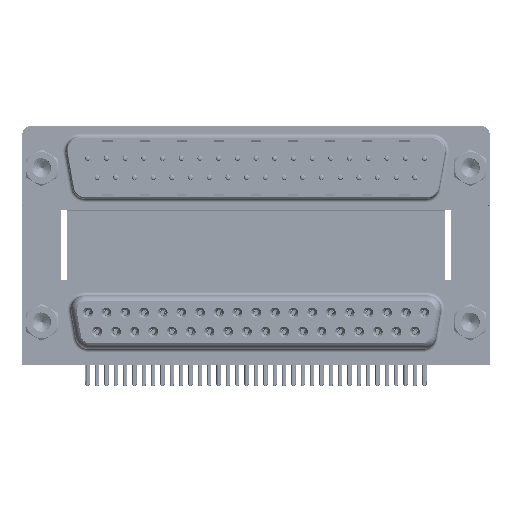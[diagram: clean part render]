
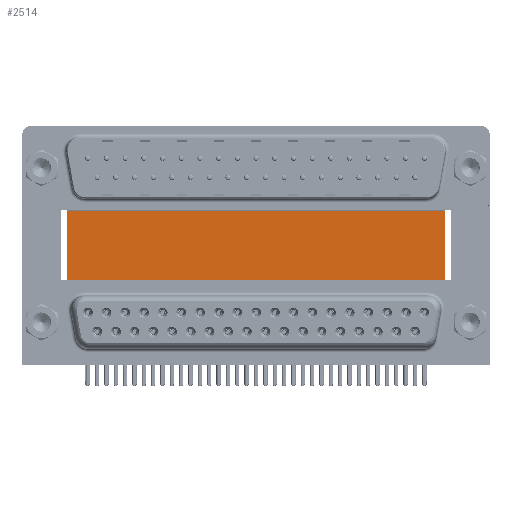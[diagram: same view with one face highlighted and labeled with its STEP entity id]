
A CAD part, top view. The second image highlights one B-rep face of the part: STEP entity #2514.
In plain terms, the highlighted planar face has unit normal (0, 0, 1).
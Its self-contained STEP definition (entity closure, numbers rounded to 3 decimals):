
#83 = VECTOR ( 'NONE', #49330, 1000. ) ;
#2514 = ADVANCED_FACE ( 'NONE', ( #45545 ), #50463, .F. ) ;
#3081 = CARTESIAN_POINT ( 'NONE',  ( 3.79, 16.585, -12. ) ) ;
#3209 = CARTESIAN_POINT ( 'NONE',  ( 3.79, 16.585, -12. ) ) ;
#4206 = DIRECTION ( 'NONE',  ( 0., 0., -1. ) ) ;
#8669 = DIRECTION ( 'NONE',  ( 1., 0., 0. ) ) ;
#8760 = LINE ( 'NONE', #3081, #83 ) ;
#18266 = CARTESIAN_POINT ( 'NONE',  ( 3.79, 16.585, -12. ) ) ;
#19559 = LINE ( 'NONE', #3209, #69572 ) ;
#19815 = VERTEX_POINT ( 'NONE', #41783 ) ;
#20115 = EDGE_CURVE ( 'NONE', #38428, #19815, #8760, .T. ) ;
#24040 = CARTESIAN_POINT ( 'NONE',  ( 59.71, 16.585, -12. ) ) ;
#29524 = EDGE_CURVE ( 'NONE', #19815, #74906, #73099, .T. ) ;
#31532 = CARTESIAN_POINT ( 'NONE',  ( 59.71, 16.585, -12. ) ) ;
#33399 = EDGE_LOOP ( 'NONE', ( #54179, #43957, #49335, #62931 ) ) ;
#38428 = VERTEX_POINT ( 'NONE', #18266 ) ;
#39738 = VERTEX_POINT ( 'NONE', #24040 ) ;
#41783 = CARTESIAN_POINT ( 'NONE',  ( 3.79, -3.735, -12. ) ) ;
#43044 = AXIS2_PLACEMENT_3D ( 'NONE', #73585, #4206, #68642 ) ;
#43837 = VECTOR ( 'NONE', #8669, 1000. ) ;
#43957 = ORIENTED_EDGE ( 'NONE', *, *, #46242, .F. ) ;
#45545 = FACE_OUTER_BOUND ( 'NONE', #33399, .T. ) ;
#46242 = EDGE_CURVE ( 'NONE', #39738, #74906, #53201, .T. ) ;
#46820 = CARTESIAN_POINT ( 'NONE',  ( 59.71, -3.735, -12. ) ) ;
#48867 = CARTESIAN_POINT ( 'NONE',  ( 3.79, -3.735, -12. ) ) ;
#49330 = DIRECTION ( 'NONE',  ( 0., -1., 0. ) ) ;
#49335 = ORIENTED_EDGE ( 'NONE', *, *, #64501, .F. ) ;
#50463 = PLANE ( 'NONE',  #43044 ) ;
#51993 = VECTOR ( 'NONE', #70634, 1000. ) ;
#53201 = LINE ( 'NONE', #31532, #51993 ) ;
#54179 = ORIENTED_EDGE ( 'NONE', *, *, #29524, .T. ) ;
#62931 = ORIENTED_EDGE ( 'NONE', *, *, #20115, .T. ) ;
#64501 = EDGE_CURVE ( 'NONE', #38428, #39738, #19559, .T. ) ;
#68642 = DIRECTION ( 'NONE',  ( -1., 0., 0. ) ) ;
#69572 = VECTOR ( 'NONE', #71841, 1000. ) ;
#70634 = DIRECTION ( 'NONE',  ( 0., -1., 0. ) ) ;
#71841 = DIRECTION ( 'NONE',  ( 1., 0., 0. ) ) ;
#73099 = LINE ( 'NONE', #48867, #43837 ) ;
#73585 = CARTESIAN_POINT ( 'NONE',  ( 3.79, 16.585, -12. ) ) ;
#74906 = VERTEX_POINT ( 'NONE', #46820 ) ;
